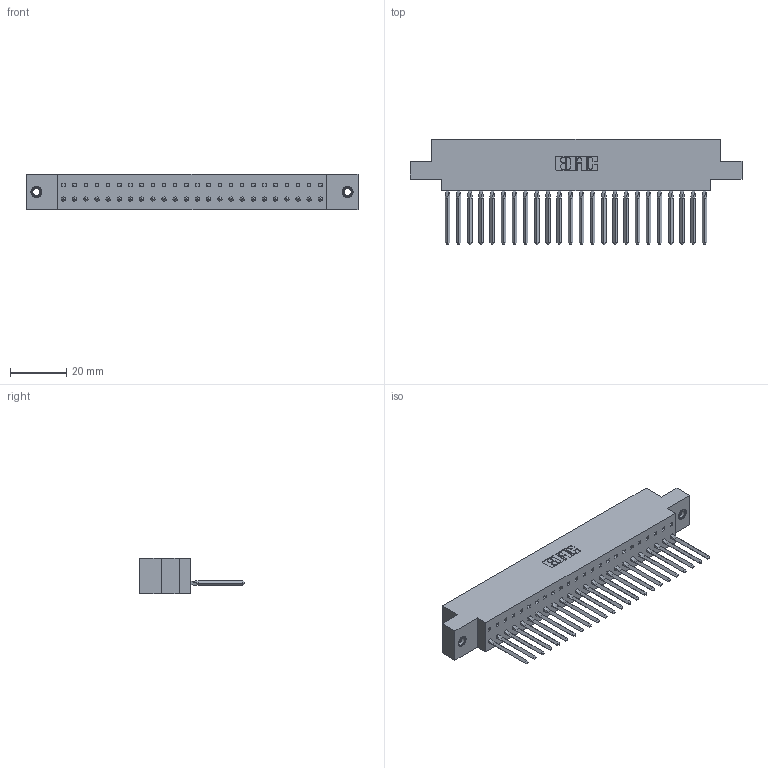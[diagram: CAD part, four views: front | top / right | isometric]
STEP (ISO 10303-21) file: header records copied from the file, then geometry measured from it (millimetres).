
FILE_DESCRIPTION (( 'STEP AP203' ), '1' );
FILE_NAME ('317-024-541-607.STEP', '2020-02-27T18:00:36', ( '' ), ( '' ), 'SwSTEP 2.0', 'SolidWorks 2016', '' );
FILE_SCHEMA (( 'CONFIG_CONTROL_DESIGN' ));
Length unit declared in the file: inch
Products named in the file (4): 317-290-002_541; 317-024-541-607; 345-250-001_345-250-005-103; 317 Part_.156 Dia - TI
Assembly tree (27 placements, depth 2):
  317-024-541-607
    317 Part_.156 Dia - TI
    317-290-002_541  x24
    345-250-001_345-250-005-103  x2
Bounding box: 117.81 x 37.34 x 12.7 mm (x, y, z)
Volume: 18537.1 mm3; surface area: 25629.5 mm2
Topology: 27 solids, 27 shells, 3810 faces, 10827 edges, 7034 vertices
Faces by surface type: plane 3066, cylinder 632, bspline 96, cone 12, torus 4
Entity records: 39169 total; most frequent: CARTESIAN_POINT 7564, ORIENTED_EDGE 6834, DIRECTION 5643, EDGE_CURVE 3417, LINE 3033, VECTOR 3033, VERTEX_POINT 2266, AXIS2_PLACEMENT_3D 1305
